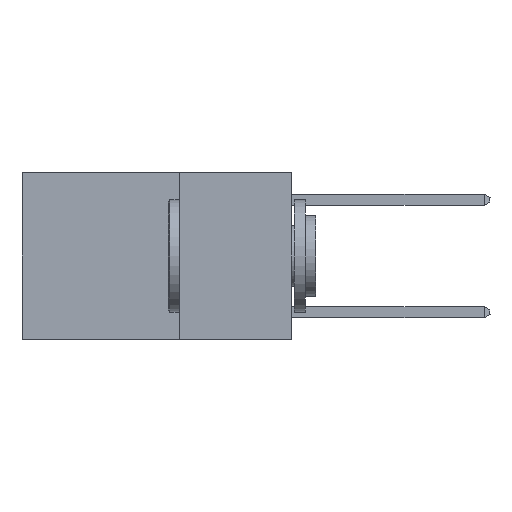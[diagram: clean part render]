
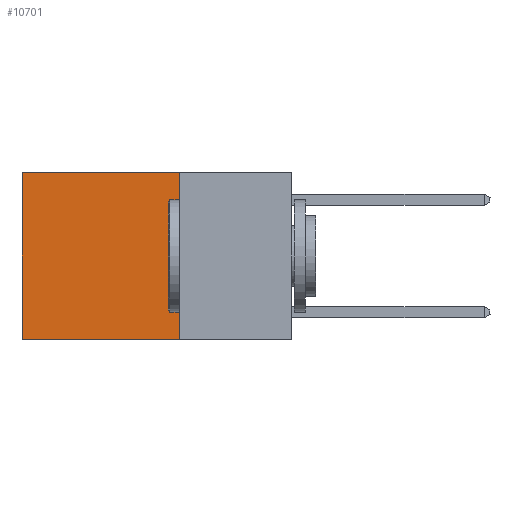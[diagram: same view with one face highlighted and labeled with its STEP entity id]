
A CAD part, left-side view. The second image highlights one B-rep face of the part: STEP entity #10701.
In plain terms, the highlighted planar face has unit normal (-1, 0, 0).
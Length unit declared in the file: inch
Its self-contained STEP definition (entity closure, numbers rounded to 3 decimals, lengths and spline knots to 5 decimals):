
#170 = VERTEX_POINT ( 'NONE', #4086 ) ;
#378 = CARTESIAN_POINT ( 'NONE',  ( 0.2625, 0.25, -0.37 ) ) ;
#761 = PLANE ( 'NONE',  #2520 ) ;
#1049 = CARTESIAN_POINT ( 'NONE',  ( 0.2625, 0.25, 0. ) ) ;
#1444 = VECTOR ( 'NONE', #9873, 39.37008 ) ;
#1729 = DIRECTION ( 'NONE',  ( 0., 0., -1. ) ) ;
#1885 = DIRECTION ( 'NONE',  ( 0., 0., -1. ) ) ;
#2461 = CARTESIAN_POINT ( 'NONE',  ( 0.2625, 0.6, 0. ) ) ;
#2520 = AXIS2_PLACEMENT_3D ( 'NONE', #9942, #9985, #1729 ) ;
#2635 = VECTOR ( 'NONE', #1885, 39.37008 ) ;
#2646 = EDGE_CURVE ( 'NONE', #11496, #3579, #11029, .T. ) ;
#3324 = DIRECTION ( 'NONE',  ( 0., 1., 0. ) ) ;
#3325 = CARTESIAN_POINT ( 'NONE',  ( 0.2625, 0.25, -0.37 ) ) ;
#3579 = VERTEX_POINT ( 'NONE', #3325 ) ;
#4029 = VERTEX_POINT ( 'NONE', #4971 ) ;
#4086 = CARTESIAN_POINT ( 'NONE',  ( 0.2625, 0.6, -0.37 ) ) ;
#4926 = EDGE_CURVE ( 'NONE', #4029, #170, #9073, .T. ) ;
#4971 = CARTESIAN_POINT ( 'NONE',  ( 0.2625, 0.6, 0. ) ) ;
#5000 = EDGE_CURVE ( 'NONE', #11496, #4029, #6523, .T. ) ;
#5561 = CARTESIAN_POINT ( 'NONE',  ( 0.2625, 0.25, 0. ) ) ;
#6449 = CARTESIAN_POINT ( 'NONE',  ( 0.2625, 0.25, 0. ) ) ;
#6523 = LINE ( 'NONE', #1049, #11620 ) ;
#7227 = FACE_OUTER_BOUND ( 'NONE', #10518, .T. ) ;
#9073 = LINE ( 'NONE', #2461, #1444 ) ;
#9110 = VECTOR ( 'NONE', #3324, 39.37008 ) ;
#9157 = ORIENTED_EDGE ( 'NONE', *, *, #5000, .T. ) ;
#9191 = EDGE_CURVE ( 'NONE', #3579, #170, #10755, .T. ) ;
#9475 = DIRECTION ( 'NONE',  ( 0., 1., 0. ) ) ;
#9873 = DIRECTION ( 'NONE',  ( 0., 0., -1. ) ) ;
#9942 = CARTESIAN_POINT ( 'NONE',  ( 0.2625, 0.25, 0. ) ) ;
#9985 = DIRECTION ( 'NONE',  ( 1., 0., 0. ) ) ;
#10328 = ORIENTED_EDGE ( 'NONE', *, *, #4926, .T. ) ;
#10518 = EDGE_LOOP ( 'NONE', ( #10328, #10754, #10563, #9157 ) ) ;
#10563 = ORIENTED_EDGE ( 'NONE', *, *, #2646, .F. ) ;
#10701 = ADVANCED_FACE ( 'NONE', ( #7227 ), #761, .F. ) ;
#10754 = ORIENTED_EDGE ( 'NONE', *, *, #9191, .F. ) ;
#10755 = LINE ( 'NONE', #378, #9110 ) ;
#11029 = LINE ( 'NONE', #6449, #2635 ) ;
#11496 = VERTEX_POINT ( 'NONE', #5561 ) ;
#11620 = VECTOR ( 'NONE', #9475, 39.37008 ) ;
